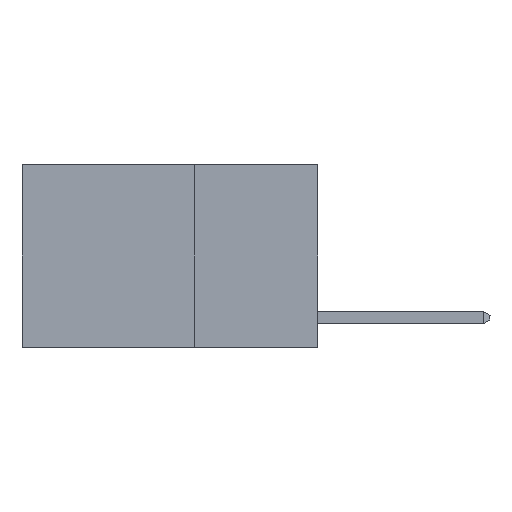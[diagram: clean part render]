
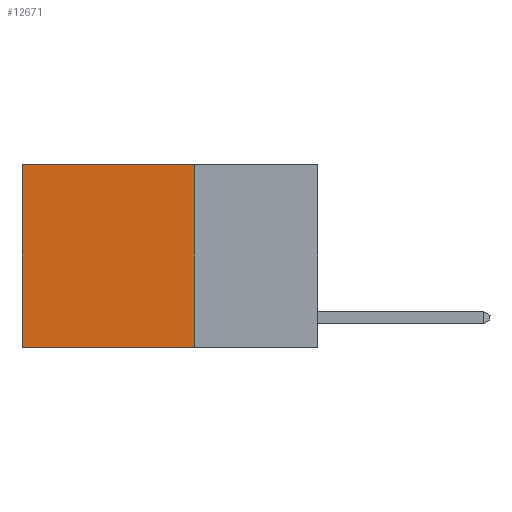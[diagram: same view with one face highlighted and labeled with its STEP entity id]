
A CAD part, left-side view. The second image highlights one B-rep face of the part: STEP entity #12671.
In plain terms, the highlighted planar face has unit normal (-1, 0, 0).
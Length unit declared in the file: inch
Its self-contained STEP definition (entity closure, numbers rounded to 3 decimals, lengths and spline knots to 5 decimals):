
#561 = CARTESIAN_POINT ( 'NONE',  ( 0.2625, 0.25, 0. ) ) ;
#799 = LINE ( 'NONE', #561, #13391 ) ;
#1980 = DIRECTION ( 'NONE',  ( 0., 0., -1. ) ) ;
#2255 = EDGE_CURVE ( 'NONE', #2587, #7556, #799, .T. ) ;
#2587 = VERTEX_POINT ( 'NONE', #8494 ) ;
#3088 = VECTOR ( 'NONE', #4346, 39.37008 ) ;
#3637 = EDGE_CURVE ( 'NONE', #2587, #11861, #9722, .T. ) ;
#4217 = EDGE_CURVE ( 'NONE', #7556, #11527, #11823, .T. ) ;
#4346 = DIRECTION ( 'NONE',  ( 0., 1., 0. ) ) ;
#5508 = ORIENTED_EDGE ( 'NONE', *, *, #2255, .F. ) ;
#5549 = CARTESIAN_POINT ( 'NONE',  ( 0.2625, 0.25, 0. ) ) ;
#6309 = EDGE_LOOP ( 'NONE', ( #7334, #12000, #5508, #13771 ) ) ;
#6665 = CARTESIAN_POINT ( 'NONE',  ( 0.2625, 0.25, -0.37 ) ) ;
#6689 = PLANE ( 'NONE',  #7734 ) ;
#6752 = VECTOR ( 'NONE', #10269, 39.37008 ) ;
#7334 = ORIENTED_EDGE ( 'NONE', *, *, #12491, .T. ) ;
#7556 = VERTEX_POINT ( 'NONE', #13694 ) ;
#7734 = AXIS2_PLACEMENT_3D ( 'NONE', #5549, #8917, #1980 ) ;
#8494 = CARTESIAN_POINT ( 'NONE',  ( 0.2625, 0.25, 0. ) ) ;
#8579 = CARTESIAN_POINT ( 'NONE',  ( 0.2625, 0.6, 0. ) ) ;
#8759 = CARTESIAN_POINT ( 'NONE',  ( 0.2625, 0.6, -0.37 ) ) ;
#8917 = DIRECTION ( 'NONE',  ( 1., 0., 0. ) ) ;
#9722 = LINE ( 'NONE', #12436, #6752 ) ;
#10021 = LINE ( 'NONE', #8579, #12963 ) ;
#10269 = DIRECTION ( 'NONE',  ( 0., 1., 0. ) ) ;
#10880 = DIRECTION ( 'NONE',  ( 0., 0., -1. ) ) ;
#11527 = VERTEX_POINT ( 'NONE', #8759 ) ;
#11823 = LINE ( 'NONE', #6665, #3088 ) ;
#11861 = VERTEX_POINT ( 'NONE', #14046 ) ;
#12000 = ORIENTED_EDGE ( 'NONE', *, *, #4217, .F. ) ;
#12436 = CARTESIAN_POINT ( 'NONE',  ( 0.2625, 0.25, 0. ) ) ;
#12491 = EDGE_CURVE ( 'NONE', #11861, #11527, #10021, .T. ) ;
#12671 = ADVANCED_FACE ( 'NONE', ( #12980 ), #6689, .F. ) ;
#12963 = VECTOR ( 'NONE', #10880, 39.37008 ) ;
#12980 = FACE_OUTER_BOUND ( 'NONE', #6309, .T. ) ;
#13391 = VECTOR ( 'NONE', #14363, 39.37008 ) ;
#13694 = CARTESIAN_POINT ( 'NONE',  ( 0.2625, 0.25, -0.37 ) ) ;
#13771 = ORIENTED_EDGE ( 'NONE', *, *, #3637, .T. ) ;
#14046 = CARTESIAN_POINT ( 'NONE',  ( 0.2625, 0.6, 0. ) ) ;
#14363 = DIRECTION ( 'NONE',  ( 0., 0., -1. ) ) ;
